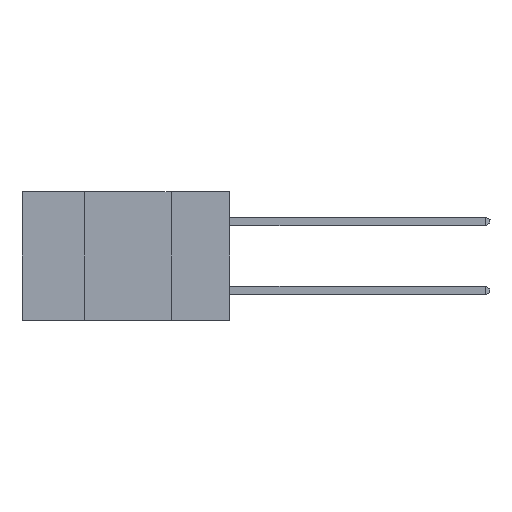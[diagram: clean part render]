
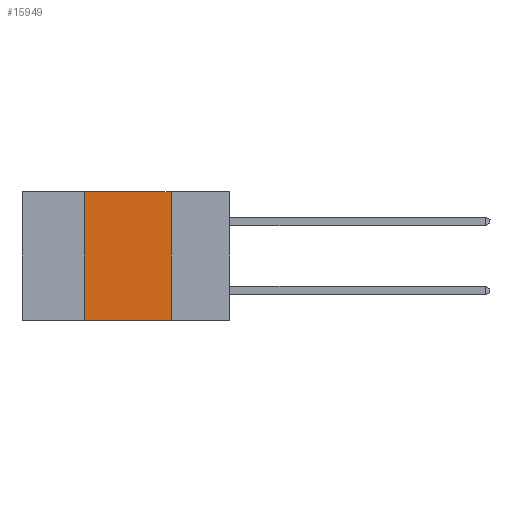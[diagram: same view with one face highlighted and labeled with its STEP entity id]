
A CAD part, left-side view. The second image highlights one B-rep face of the part: STEP entity #15949.
In plain terms, the highlighted planar face has unit normal (-1, 0, 0).
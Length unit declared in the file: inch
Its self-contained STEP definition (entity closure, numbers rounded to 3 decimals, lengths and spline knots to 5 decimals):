
#18 = LINE ( 'NONE', #14830, #2266 ) ;
#455 = DIRECTION ( 'NONE',  ( 0., -1., 0. ) ) ;
#2116 = FACE_OUTER_BOUND ( 'NONE', #5150, .T. ) ;
#2266 = VECTOR ( 'NONE', #455, 39.37008 ) ;
#2956 = VECTOR ( 'NONE', #7053, 39.37008 ) ;
#3205 = EDGE_CURVE ( 'NONE', #11871, #14366, #5939, .T. ) ;
#3272 = CARTESIAN_POINT ( 'NONE',  ( 0., 0.17, 0. ) ) ;
#3785 = ORIENTED_EDGE ( 'NONE', *, *, #5970, .T. ) ;
#5150 = EDGE_LOOP ( 'NONE', ( #11041, #11900, #6191, #3785 ) ) ;
#5925 = LINE ( 'NONE', #3272, #7157 ) ;
#5939 = LINE ( 'NONE', #6336, #7582 ) ;
#5970 = EDGE_CURVE ( 'NONE', #11871, #11845, #6447, .T. ) ;
#6191 = ORIENTED_EDGE ( 'NONE', *, *, #3205, .F. ) ;
#6336 = CARTESIAN_POINT ( 'NONE',  ( 0., 0.42, 0. ) ) ;
#6447 = LINE ( 'NONE', #15086, #2956 ) ;
#7053 = DIRECTION ( 'NONE',  ( 0., -1., 0. ) ) ;
#7157 = VECTOR ( 'NONE', #8604, 39.37008 ) ;
#7494 = VERTEX_POINT ( 'NONE', #16758 ) ;
#7582 = VECTOR ( 'NONE', #14282, 39.37008 ) ;
#7615 = DIRECTION ( 'NONE',  ( 1., 0., 0. ) ) ;
#8604 = DIRECTION ( 'NONE',  ( 0., 0., -1. ) ) ;
#9642 = EDGE_CURVE ( 'NONE', #7494, #11845, #5925, .T. ) ;
#10247 = DIRECTION ( 'NONE',  ( 0., 0., -1. ) ) ;
#10751 = CARTESIAN_POINT ( 'NONE',  ( 0., 0.42, -0.37 ) ) ;
#11041 = ORIENTED_EDGE ( 'NONE', *, *, #9642, .F. ) ;
#11845 = VERTEX_POINT ( 'NONE', #11861 ) ;
#11861 = CARTESIAN_POINT ( 'NONE',  ( 0., 0.17, -0.37 ) ) ;
#11871 = VERTEX_POINT ( 'NONE', #10751 ) ;
#11876 = EDGE_CURVE ( 'NONE', #14366, #7494, #18, .T. ) ;
#11900 = ORIENTED_EDGE ( 'NONE', *, *, #11876, .F. ) ;
#12021 = CARTESIAN_POINT ( 'NONE',  ( 0., 0.42, 0. ) ) ;
#12948 = CARTESIAN_POINT ( 'NONE',  ( 0., 0.6, 0. ) ) ;
#14282 = DIRECTION ( 'NONE',  ( 0., 0., 1. ) ) ;
#14366 = VERTEX_POINT ( 'NONE', #12021 ) ;
#14830 = CARTESIAN_POINT ( 'NONE',  ( 0., 0.6, 0. ) ) ;
#15086 = CARTESIAN_POINT ( 'NONE',  ( 0., 0.6, -0.37 ) ) ;
#15497 = PLANE ( 'NONE',  #15563 ) ;
#15563 = AXIS2_PLACEMENT_3D ( 'NONE', #12948, #7615, #10247 ) ;
#15949 = ADVANCED_FACE ( 'NONE', ( #2116 ), #15497, .F. ) ;
#16758 = CARTESIAN_POINT ( 'NONE',  ( 0., 0.17, 0. ) ) ;
